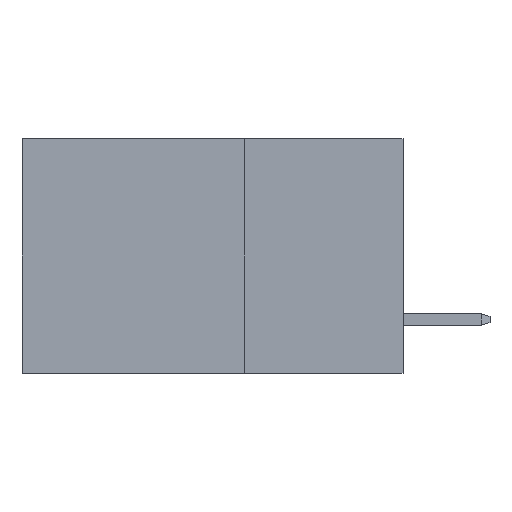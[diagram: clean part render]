
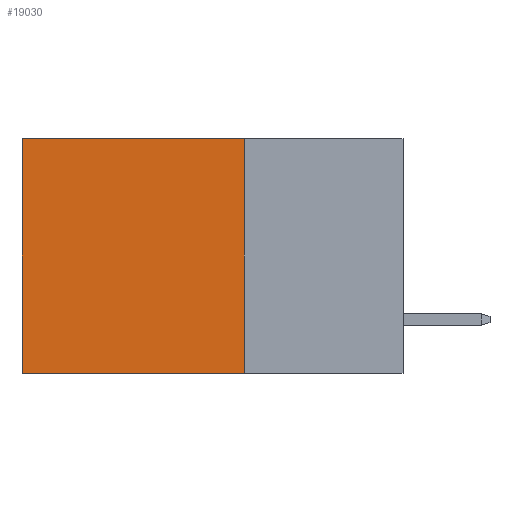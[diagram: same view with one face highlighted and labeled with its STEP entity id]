
A CAD part, left-side view. The second image highlights one B-rep face of the part: STEP entity #19030.
In plain terms, the highlighted planar face has unit normal (-1, 0, 0).
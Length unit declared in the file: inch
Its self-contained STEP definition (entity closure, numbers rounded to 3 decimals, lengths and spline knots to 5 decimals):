
#255 = CARTESIAN_POINT ( 'NONE',  ( 0.2875, 0.25, 0. ) ) ;
#1114 = CARTESIAN_POINT ( 'NONE',  ( 0.2875, 0.6, 0. ) ) ;
#1596 = CARTESIAN_POINT ( 'NONE',  ( 0.2875, 0.6, 0. ) ) ;
#2693 = EDGE_CURVE ( 'NONE', #4694, #6907, #7923, .T. ) ;
#3766 = CARTESIAN_POINT ( 'NONE',  ( 0.2875, 0.6, -0.37 ) ) ;
#4327 = DIRECTION ( 'NONE',  ( 0., 0., -1. ) ) ;
#4694 = VERTEX_POINT ( 'NONE', #9822 ) ;
#5235 = DIRECTION ( 'NONE',  ( 0., 0., -1. ) ) ;
#5238 = VECTOR ( 'NONE', #4327, 39.37008 ) ;
#5665 = CARTESIAN_POINT ( 'NONE',  ( 0.2875, 0.25, 0. ) ) ;
#6907 = VERTEX_POINT ( 'NONE', #1114 ) ;
#7190 = ORIENTED_EDGE ( 'NONE', *, *, #25857, .F. ) ;
#7646 = VERTEX_POINT ( 'NONE', #13730 ) ;
#7923 = LINE ( 'NONE', #5665, #21101 ) ;
#8162 = LINE ( 'NONE', #23714, #15082 ) ;
#8842 = LINE ( 'NONE', #1596, #5238 ) ;
#9173 = VERTEX_POINT ( 'NONE', #3766 ) ;
#9176 = ORIENTED_EDGE ( 'NONE', *, *, #2693, .T. ) ;
#9822 = CARTESIAN_POINT ( 'NONE',  ( 0.2875, 0.25, 0. ) ) ;
#9892 = AXIS2_PLACEMENT_3D ( 'NONE', #255, #25927, #5235 ) ;
#10921 = VECTOR ( 'NONE', #21508, 39.37008 ) ;
#11299 = EDGE_CURVE ( 'NONE', #6907, #9173, #8842, .T. ) ;
#13529 = ORIENTED_EDGE ( 'NONE', *, *, #11299, .T. ) ;
#13730 = CARTESIAN_POINT ( 'NONE',  ( 0.2875, 0.25, -0.37 ) ) ;
#14885 = DIRECTION ( 'NONE',  ( 0., 1., 0. ) ) ;
#15082 = VECTOR ( 'NONE', #21306, 39.37008 ) ;
#15794 = EDGE_CURVE ( 'NONE', #4694, #7646, #8162, .T. ) ;
#17111 = LINE ( 'NONE', #19251, #10921 ) ;
#19030 = ADVANCED_FACE ( 'NONE', ( #20939 ), #25630, .F. ) ;
#19251 = CARTESIAN_POINT ( 'NONE',  ( 0.2875, 0.25, -0.37 ) ) ;
#20236 = ORIENTED_EDGE ( 'NONE', *, *, #15794, .F. ) ;
#20939 = FACE_OUTER_BOUND ( 'NONE', #23547, .T. ) ;
#21101 = VECTOR ( 'NONE', #14885, 39.37008 ) ;
#21306 = DIRECTION ( 'NONE',  ( 0., 0., -1. ) ) ;
#21508 = DIRECTION ( 'NONE',  ( 0., 1., 0. ) ) ;
#23547 = EDGE_LOOP ( 'NONE', ( #13529, #7190, #20236, #9176 ) ) ;
#23714 = CARTESIAN_POINT ( 'NONE',  ( 0.2875, 0.25, 0. ) ) ;
#25630 = PLANE ( 'NONE',  #9892 ) ;
#25857 = EDGE_CURVE ( 'NONE', #7646, #9173, #17111, .T. ) ;
#25927 = DIRECTION ( 'NONE',  ( 1., 0., 0. ) ) ;
